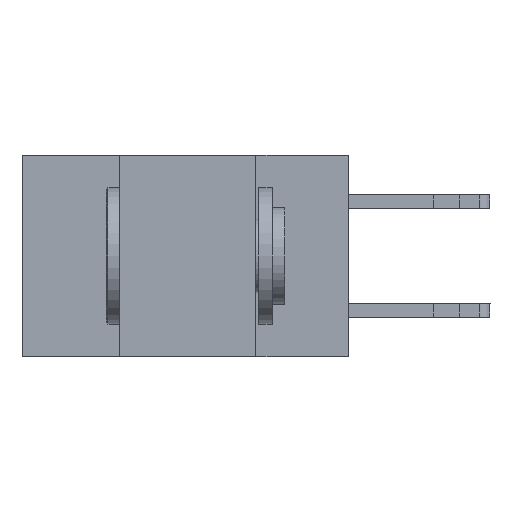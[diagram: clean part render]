
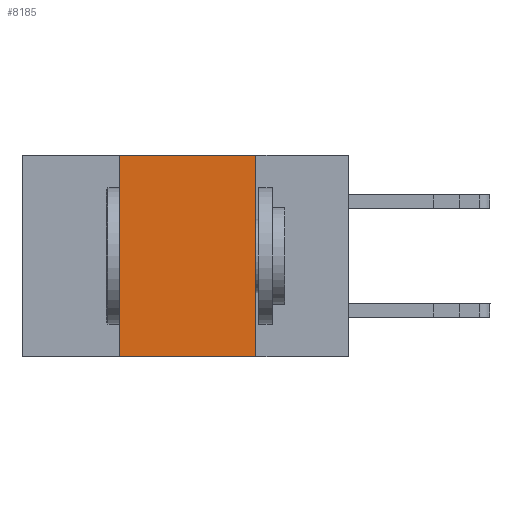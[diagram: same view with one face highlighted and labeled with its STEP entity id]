
A CAD part, left-side view. The second image highlights one B-rep face of the part: STEP entity #8185.
In plain terms, the highlighted planar face has unit normal (-1, 0, 0).
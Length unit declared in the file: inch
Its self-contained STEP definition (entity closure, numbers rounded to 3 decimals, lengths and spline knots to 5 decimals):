
#1058 = CARTESIAN_POINT ( 'NONE',  ( 0., 0.17, 0. ) ) ;
#1319 = ORIENTED_EDGE ( 'NONE', *, *, #5491, .F. ) ;
#1422 = CARTESIAN_POINT ( 'NONE',  ( 0., 0.6, -0.37 ) ) ;
#1576 = FACE_OUTER_BOUND ( 'NONE', #6584, .T. ) ;
#1586 = DIRECTION ( 'NONE',  ( 0., -1., 0. ) ) ;
#1640 = ORIENTED_EDGE ( 'NONE', *, *, #5682, .T. ) ;
#1881 = CARTESIAN_POINT ( 'NONE',  ( 0., 0.42, 0. ) ) ;
#1994 = LINE ( 'NONE', #12077, #3185 ) ;
#2445 = VERTEX_POINT ( 'NONE', #1058 ) ;
#2462 = LINE ( 'NONE', #12207, #12083 ) ;
#3163 = VECTOR ( 'NONE', #6728, 39.37008 ) ;
#3185 = VECTOR ( 'NONE', #9066, 39.37008 ) ;
#3985 = VERTEX_POINT ( 'NONE', #8468 ) ;
#4060 = VECTOR ( 'NONE', #1586, 39.37008 ) ;
#5028 = DIRECTION ( 'NONE',  ( 1., 0., 0. ) ) ;
#5491 = EDGE_CURVE ( 'NONE', #3985, #6409, #7999, .T. ) ;
#5552 = LINE ( 'NONE', #1422, #4060 ) ;
#5641 = AXIS2_PLACEMENT_3D ( 'NONE', #7079, #5028, #10393 ) ;
#5682 = EDGE_CURVE ( 'NONE', #3985, #5903, #5552, .T. ) ;
#5800 = ORIENTED_EDGE ( 'NONE', *, *, #9564, .F. ) ;
#5903 = VERTEX_POINT ( 'NONE', #11688 ) ;
#6306 = DIRECTION ( 'NONE',  ( 0., -1., 0. ) ) ;
#6409 = VERTEX_POINT ( 'NONE', #1881 ) ;
#6509 = CARTESIAN_POINT ( 'NONE',  ( 0., 0.42, 0. ) ) ;
#6584 = EDGE_LOOP ( 'NONE', ( #8674, #5800, #1319, #1640 ) ) ;
#6728 = DIRECTION ( 'NONE',  ( 0., 0., 1. ) ) ;
#7079 = CARTESIAN_POINT ( 'NONE',  ( 0., 0.6, 0. ) ) ;
#7120 = PLANE ( 'NONE',  #5641 ) ;
#7999 = LINE ( 'NONE', #6509, #3163 ) ;
#8185 = ADVANCED_FACE ( 'NONE', ( #1576 ), #7120, .F. ) ;
#8468 = CARTESIAN_POINT ( 'NONE',  ( 0., 0.42, -0.37 ) ) ;
#8674 = ORIENTED_EDGE ( 'NONE', *, *, #11278, .F. ) ;
#9066 = DIRECTION ( 'NONE',  ( 0., 0., -1. ) ) ;
#9564 = EDGE_CURVE ( 'NONE', #6409, #2445, #2462, .T. ) ;
#10393 = DIRECTION ( 'NONE',  ( 0., 0., -1. ) ) ;
#11278 = EDGE_CURVE ( 'NONE', #2445, #5903, #1994, .T. ) ;
#11688 = CARTESIAN_POINT ( 'NONE',  ( 0., 0.17, -0.37 ) ) ;
#12077 = CARTESIAN_POINT ( 'NONE',  ( 0., 0.17, 0. ) ) ;
#12083 = VECTOR ( 'NONE', #6306, 39.37008 ) ;
#12207 = CARTESIAN_POINT ( 'NONE',  ( 0., 0.6, 0. ) ) ;
